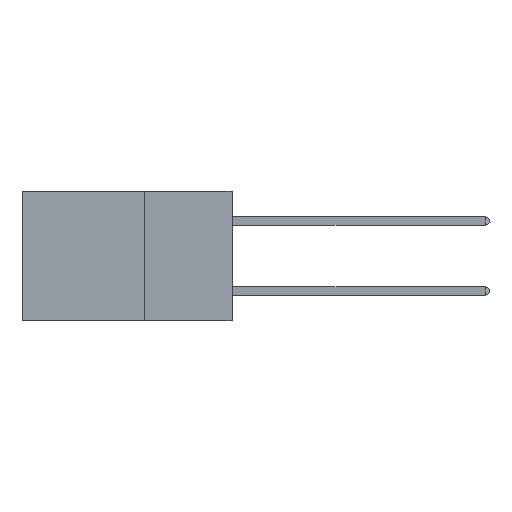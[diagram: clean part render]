
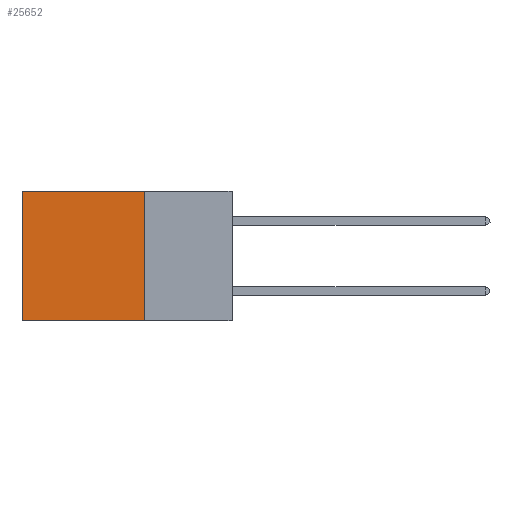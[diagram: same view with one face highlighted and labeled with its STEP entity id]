
A CAD part, left-side view. The second image highlights one B-rep face of the part: STEP entity #25652.
In plain terms, the highlighted planar face has unit normal (-1, 0, 0).
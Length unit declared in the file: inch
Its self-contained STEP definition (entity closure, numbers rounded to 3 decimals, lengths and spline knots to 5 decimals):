
#1197 = CARTESIAN_POINT ( 'NONE',  ( 0.2875, 0.25, 0. ) ) ;
#1466 = CARTESIAN_POINT ( 'NONE',  ( 0.2875, 0.25, 0. ) ) ;
#2781 = VERTEX_POINT ( 'NONE', #26749 ) ;
#3089 = LINE ( 'NONE', #1197, #34968 ) ;
#5542 = EDGE_CURVE ( 'NONE', #30757, #37845, #27584, .T. ) ;
#6929 = VERTEX_POINT ( 'NONE', #27388 ) ;
#6958 = ORIENTED_EDGE ( 'NONE', *, *, #21478, .T. ) ;
#7652 = DIRECTION ( 'NONE',  ( 1., 0., 0. ) ) ;
#9178 = CARTESIAN_POINT ( 'NONE',  ( 0.2875, 0.25, -0.37 ) ) ;
#9335 = EDGE_CURVE ( 'NONE', #2781, #37845, #37004, .T. ) ;
#11530 = VECTOR ( 'NONE', #38897, 39.37008 ) ;
#11571 = LINE ( 'NONE', #22148, #35579 ) ;
#15031 = ORIENTED_EDGE ( 'NONE', *, *, #5542, .F. ) ;
#16643 = EDGE_LOOP ( 'NONE', ( #21194, #15031, #38559, #6958 ) ) ;
#20107 = DIRECTION ( 'NONE',  ( 0., 0., -1. ) ) ;
#21194 = ORIENTED_EDGE ( 'NONE', *, *, #9335, .T. ) ;
#21478 = EDGE_CURVE ( 'NONE', #6929, #2781, #11571, .T. ) ;
#22148 = CARTESIAN_POINT ( 'NONE',  ( 0.2875, 0.25, 0. ) ) ;
#23012 = EDGE_CURVE ( 'NONE', #6929, #30757, #3089, .T. ) ;
#24511 = CARTESIAN_POINT ( 'NONE',  ( 0.2875, 0.6, -0.37 ) ) ;
#25652 = ADVANCED_FACE ( 'NONE', ( #35253 ), #26167, .F. ) ;
#25845 = DIRECTION ( 'NONE',  ( 0., 1., 0. ) ) ;
#26167 = PLANE ( 'NONE',  #33955 ) ;
#26749 = CARTESIAN_POINT ( 'NONE',  ( 0.2875, 0.6, 0. ) ) ;
#27388 = CARTESIAN_POINT ( 'NONE',  ( 0.2875, 0.25, 0. ) ) ;
#27584 = LINE ( 'NONE', #29461, #39835 ) ;
#29461 = CARTESIAN_POINT ( 'NONE',  ( 0.2875, 0.25, -0.37 ) ) ;
#30757 = VERTEX_POINT ( 'NONE', #9178 ) ;
#32599 = DIRECTION ( 'NONE',  ( 0., 1., 0. ) ) ;
#32876 = DIRECTION ( 'NONE',  ( 0., 0., -1. ) ) ;
#33955 = AXIS2_PLACEMENT_3D ( 'NONE', #1466, #7652, #32876 ) ;
#34968 = VECTOR ( 'NONE', #20107, 39.37008 ) ;
#35253 = FACE_OUTER_BOUND ( 'NONE', #16643, .T. ) ;
#35579 = VECTOR ( 'NONE', #25845, 39.37008 ) ;
#35885 = CARTESIAN_POINT ( 'NONE',  ( 0.2875, 0.6, 0. ) ) ;
#37004 = LINE ( 'NONE', #35885, #11530 ) ;
#37845 = VERTEX_POINT ( 'NONE', #24511 ) ;
#38559 = ORIENTED_EDGE ( 'NONE', *, *, #23012, .F. ) ;
#38897 = DIRECTION ( 'NONE',  ( 0., 0., -1. ) ) ;
#39835 = VECTOR ( 'NONE', #32599, 39.37008 ) ;
